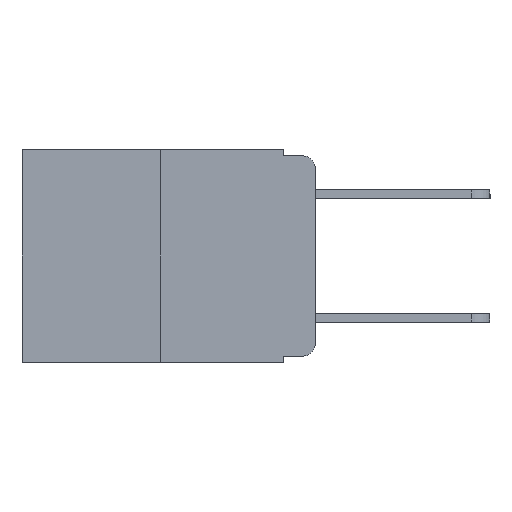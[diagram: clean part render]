
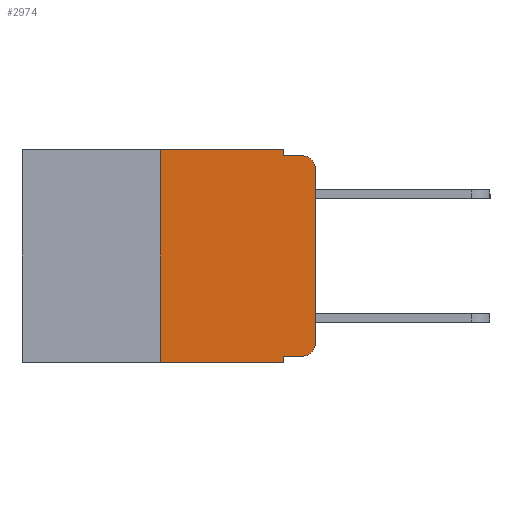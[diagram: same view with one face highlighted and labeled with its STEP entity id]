
A CAD part, left-side view. The second image highlights one B-rep face of the part: STEP entity #2974.
In plain terms, the highlighted planar face has unit normal (-1, 0, 0).
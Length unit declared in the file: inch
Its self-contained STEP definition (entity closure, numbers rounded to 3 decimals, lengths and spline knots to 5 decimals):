
#73 = ORIENTED_EDGE ( 'NONE', *, *, #13843, .T. ) ;
#337 = EDGE_CURVE ( 'NONE', #13966, #5687, #13701, .T. ) ;
#426 = LINE ( 'NONE', #11781, #3431 ) ;
#521 = ORIENTED_EDGE ( 'NONE', *, *, #13148, .T. ) ;
#745 = ORIENTED_EDGE ( 'NONE', *, *, #6312, .T. ) ;
#760 = DIRECTION ( 'NONE',  ( 0., -1., 0. ) ) ;
#801 = CARTESIAN_POINT ( 'NONE',  ( 0., 0.051, 0. ) ) ;
#817 = CARTESIAN_POINT ( 'NONE',  ( 0., 0.051, -0.333 ) ) ;
#954 = LINE ( 'NONE', #5876, #13080 ) ;
#1241 = DIRECTION ( 'NONE',  ( 0., 0., 1. ) ) ;
#1488 = CARTESIAN_POINT ( 'NONE',  ( 0., 0.473, 0. ) ) ;
#1688 = VERTEX_POINT ( 'NONE', #4499 ) ;
#1794 = CIRCLE ( 'NONE', #8280, 0.02 ) ;
#1798 = EDGE_CURVE ( 'NONE', #11003, #4148, #10099, .T. ) ;
#2120 = VECTOR ( 'NONE', #1241, 39.37008 ) ;
#2165 = VECTOR ( 'NONE', #5809, 39.37008 ) ;
#2373 = CIRCLE ( 'NONE', #11468, 0.02 ) ;
#2387 = VERTEX_POINT ( 'NONE', #3807 ) ;
#2403 = DIRECTION ( 'NONE',  ( 0., -1., 0. ) ) ;
#2974 = ADVANCED_FACE ( 'NONE', ( #6833 ), #9554, .F. ) ;
#3173 = CARTESIAN_POINT ( 'NONE',  ( 0., 0.25, -0.343 ) ) ;
#3431 = VECTOR ( 'NONE', #12818, 39.37008 ) ;
#3669 = ORIENTED_EDGE ( 'NONE', *, *, #1798, .T. ) ;
#3807 = CARTESIAN_POINT ( 'NONE',  ( 0., 0.051, -0.343 ) ) ;
#4148 = VERTEX_POINT ( 'NONE', #4722 ) ;
#4499 = CARTESIAN_POINT ( 'NONE',  ( 0., 0., -0.03 ) ) ;
#4722 = CARTESIAN_POINT ( 'NONE',  ( 0., 0.02, -0.333 ) ) ;
#4959 = EDGE_LOOP ( 'NONE', ( #73, #521, #8698, #13514, #9934, #10572, #745, #12838, #3669, #13391 ) ) ;
#5025 = CARTESIAN_POINT ( 'NONE',  ( 0., 0.02, -0.03 ) ) ;
#5268 = CARTESIAN_POINT ( 'NONE',  ( 0., 0.02, -0.313 ) ) ;
#5436 = LINE ( 'NONE', #801, #2165 ) ;
#5687 = VERTEX_POINT ( 'NONE', #14498 ) ;
#5809 = DIRECTION ( 'NONE',  ( 0., 0., -1. ) ) ;
#5876 = CARTESIAN_POINT ( 'NONE',  ( 0., 0., 0. ) ) ;
#6197 = DIRECTION ( 'NONE',  ( 0., 0., -1. ) ) ;
#6262 = AXIS2_PLACEMENT_3D ( 'NONE', #8388, #13142, #8315 ) ;
#6312 = EDGE_CURVE ( 'NONE', #13655, #2387, #13413, .T. ) ;
#6446 = DIRECTION ( 'NONE',  ( 0., 0., -1. ) ) ;
#6721 = EDGE_CURVE ( 'NONE', #11003, #2387, #5436, .T. ) ;
#6833 = FACE_OUTER_BOUND ( 'NONE', #4959, .T. ) ;
#7251 = CARTESIAN_POINT ( 'NONE',  ( 0., 0.051, -0.01 ) ) ;
#8129 = VECTOR ( 'NONE', #2403, 39.37008 ) ;
#8195 = VECTOR ( 'NONE', #14507, 39.37008 ) ;
#8280 = AXIS2_PLACEMENT_3D ( 'NONE', #5025, #12641, #6197 ) ;
#8305 = EDGE_CURVE ( 'NONE', #13655, #13966, #14006, .T. ) ;
#8315 = DIRECTION ( 'NONE',  ( 0., 0., -1. ) ) ;
#8340 = CARTESIAN_POINT ( 'NONE',  ( 0., 0.051, -0.01 ) ) ;
#8388 = CARTESIAN_POINT ( 'NONE',  ( 0., 0.473, 0. ) ) ;
#8698 = ORIENTED_EDGE ( 'NONE', *, *, #10406, .F. ) ;
#9298 = DIRECTION ( 'NONE',  ( 0., 0., 1. ) ) ;
#9346 = CARTESIAN_POINT ( 'NONE',  ( 0., 0.02, -0.01 ) ) ;
#9554 = PLANE ( 'NONE',  #6262 ) ;
#9596 = CARTESIAN_POINT ( 'NONE',  ( 0., 0.25, 0. ) ) ;
#9710 = EDGE_CURVE ( 'NONE', #5687, #11881, #426, .T. ) ;
#9934 = ORIENTED_EDGE ( 'NONE', *, *, #337, .F. ) ;
#10099 = LINE ( 'NONE', #817, #12498 ) ;
#10406 = EDGE_CURVE ( 'NONE', #11881, #13890, #13965, .T. ) ;
#10572 = ORIENTED_EDGE ( 'NONE', *, *, #8305, .F. ) ;
#10721 = CARTESIAN_POINT ( 'NONE',  ( 0., 0.473, -0.343 ) ) ;
#11003 = VERTEX_POINT ( 'NONE', #12342 ) ;
#11137 = DIRECTION ( 'NONE',  ( 0., -1., 0. ) ) ;
#11468 = AXIS2_PLACEMENT_3D ( 'NONE', #5268, #12853, #6446 ) ;
#11761 = VERTEX_POINT ( 'NONE', #12279 ) ;
#11781 = CARTESIAN_POINT ( 'NONE',  ( 0., 0.051, 0. ) ) ;
#11881 = VERTEX_POINT ( 'NONE', #8340 ) ;
#12279 = CARTESIAN_POINT ( 'NONE',  ( 0., 0., -0.313 ) ) ;
#12342 = CARTESIAN_POINT ( 'NONE',  ( 0., 0.051, -0.333 ) ) ;
#12498 = VECTOR ( 'NONE', #760, 39.37008 ) ;
#12641 = DIRECTION ( 'NONE',  ( -1., 0., 0. ) ) ;
#12818 = DIRECTION ( 'NONE',  ( 0., 0., -1. ) ) ;
#12838 = ORIENTED_EDGE ( 'NONE', *, *, #6721, .F. ) ;
#12853 = DIRECTION ( 'NONE',  ( -1., 0., 0. ) ) ;
#13068 = VECTOR ( 'NONE', #11137, 39.37008 ) ;
#13080 = VECTOR ( 'NONE', #9298, 39.37008 ) ;
#13142 = DIRECTION ( 'NONE',  ( 1., 0., 0. ) ) ;
#13148 = EDGE_CURVE ( 'NONE', #1688, #13890, #1794, .T. ) ;
#13391 = ORIENTED_EDGE ( 'NONE', *, *, #14099, .T. ) ;
#13413 = LINE ( 'NONE', #10721, #13068 ) ;
#13514 = ORIENTED_EDGE ( 'NONE', *, *, #9710, .F. ) ;
#13561 = CARTESIAN_POINT ( 'NONE',  ( 0., 0.25, 0. ) ) ;
#13655 = VERTEX_POINT ( 'NONE', #3173 ) ;
#13701 = LINE ( 'NONE', #1488, #8195 ) ;
#13843 = EDGE_CURVE ( 'NONE', #11761, #1688, #954, .T. ) ;
#13890 = VERTEX_POINT ( 'NONE', #9346 ) ;
#13965 = LINE ( 'NONE', #7251, #8129 ) ;
#13966 = VERTEX_POINT ( 'NONE', #13561 ) ;
#14006 = LINE ( 'NONE', #9596, #2120 ) ;
#14099 = EDGE_CURVE ( 'NONE', #4148, #11761, #2373, .T. ) ;
#14498 = CARTESIAN_POINT ( 'NONE',  ( 0., 0.051, 0. ) ) ;
#14507 = DIRECTION ( 'NONE',  ( 0., -1., 0. ) ) ;
